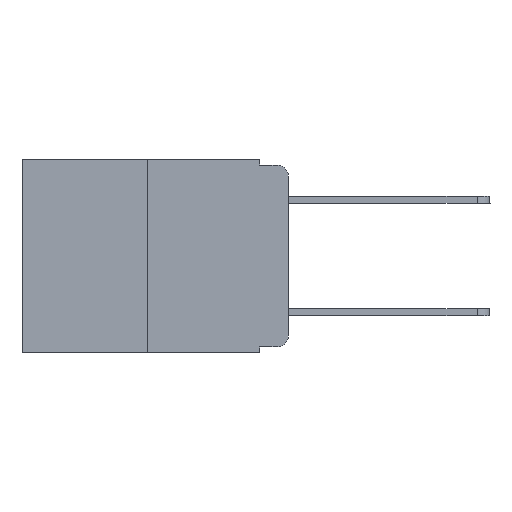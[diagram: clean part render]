
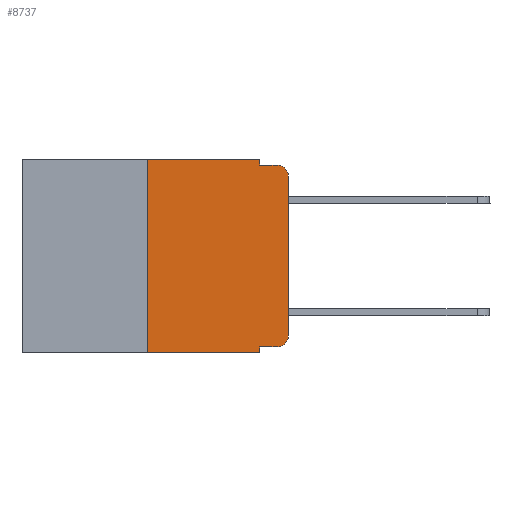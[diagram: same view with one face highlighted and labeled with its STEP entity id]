
A CAD part, left-side view. The second image highlights one B-rep face of the part: STEP entity #8737.
In plain terms, the highlighted planar face has unit normal (-1, 0, 0).
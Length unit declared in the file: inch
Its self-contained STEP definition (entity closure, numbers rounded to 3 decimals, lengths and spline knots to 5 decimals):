
#845 = VERTEX_POINT ( 'NONE', #11246 ) ;
#1171 = EDGE_CURVE ( 'NONE', #12638, #16427, #18027, .T. ) ;
#1234 = EDGE_LOOP ( 'NONE', ( #3642, #6258, #17598, #10603, #13223, #4918, #3690, #18426, #12828, #8802 ) ) ;
#1273 = VERTEX_POINT ( 'NONE', #2301 ) ;
#1366 = VECTOR ( 'NONE', #17903, 39.37008 ) ;
#1496 = DIRECTION ( 'NONE',  ( 0., -1., 0. ) ) ;
#2004 = DIRECTION ( 'NONE',  ( 0., 0., 1. ) ) ;
#2301 = CARTESIAN_POINT ( 'NONE',  ( 0., 0.051, -0.343 ) ) ;
#3559 = VECTOR ( 'NONE', #6143, 39.37008 ) ;
#3642 = ORIENTED_EDGE ( 'NONE', *, *, #10193, .T. ) ;
#3690 = ORIENTED_EDGE ( 'NONE', *, *, #9204, .T. ) ;
#3753 = DIRECTION ( 'NONE',  ( 1., 0., 0. ) ) ;
#3826 = CARTESIAN_POINT ( 'NONE',  ( 0., 0.051, -0.333 ) ) ;
#4065 = DIRECTION ( 'NONE',  ( 0., 0., 1. ) ) ;
#4355 = CARTESIAN_POINT ( 'NONE',  ( 0., 0.02, -0.333 ) ) ;
#4918 = ORIENTED_EDGE ( 'NONE', *, *, #5948, .F. ) ;
#5198 = VERTEX_POINT ( 'NONE', #15823 ) ;
#5510 = VECTOR ( 'NONE', #7941, 39.37008 ) ;
#5948 = EDGE_CURVE ( 'NONE', #6096, #845, #6166, .T. ) ;
#6059 = CARTESIAN_POINT ( 'NONE',  ( 0., 0.051, -0.01 ) ) ;
#6093 = LINE ( 'NONE', #22038, #20077 ) ;
#6096 = VERTEX_POINT ( 'NONE', #6820 ) ;
#6143 = DIRECTION ( 'NONE',  ( 0., -1., 0. ) ) ;
#6166 = LINE ( 'NONE', #13806, #19857 ) ;
#6224 = CARTESIAN_POINT ( 'NONE',  ( 0., 0.051, 0. ) ) ;
#6237 = VERTEX_POINT ( 'NONE', #18385 ) ;
#6258 = ORIENTED_EDGE ( 'NONE', *, *, #21235, .T. ) ;
#6820 = CARTESIAN_POINT ( 'NONE',  ( 0., 0.25, -0.343 ) ) ;
#7347 = VECTOR ( 'NONE', #13182, 39.37008 ) ;
#7941 = DIRECTION ( 'NONE',  ( 0., 0., -1. ) ) ;
#8374 = VERTEX_POINT ( 'NONE', #14708 ) ;
#8737 = ADVANCED_FACE ( 'NONE', ( #10487 ), #11644, .F. ) ;
#8802 = ORIENTED_EDGE ( 'NONE', *, *, #1171, .T. ) ;
#9015 = CARTESIAN_POINT ( 'NONE',  ( 0., 0.02, -0.313 ) ) ;
#9204 = EDGE_CURVE ( 'NONE', #6096, #1273, #18275, .T. ) ;
#9971 = VECTOR ( 'NONE', #1496, 39.37008 ) ;
#10018 = CARTESIAN_POINT ( 'NONE',  ( 0., 0.051, 0. ) ) ;
#10193 = EDGE_CURVE ( 'NONE', #16427, #21593, #6093, .T. ) ;
#10400 = LINE ( 'NONE', #3826, #1366 ) ;
#10487 = FACE_OUTER_BOUND ( 'NONE', #1234, .T. ) ;
#10603 = ORIENTED_EDGE ( 'NONE', *, *, #12432, .F. ) ;
#11202 = EDGE_CURVE ( 'NONE', #8374, #12638, #10400, .T. ) ;
#11246 = CARTESIAN_POINT ( 'NONE',  ( 0., 0.25, 0. ) ) ;
#11427 = CARTESIAN_POINT ( 'NONE',  ( 0., 0., -0.313 ) ) ;
#11644 = PLANE ( 'NONE',  #25113 ) ;
#12304 = DIRECTION ( 'NONE',  ( -1., 0., 0. ) ) ;
#12432 = EDGE_CURVE ( 'NONE', #24464, #6237, #25014, .T. ) ;
#12638 = VERTEX_POINT ( 'NONE', #4355 ) ;
#12828 = ORIENTED_EDGE ( 'NONE', *, *, #11202, .T. ) ;
#13182 = DIRECTION ( 'NONE',  ( 0., -1., 0. ) ) ;
#13223 = ORIENTED_EDGE ( 'NONE', *, *, #13589, .F. ) ;
#13589 = EDGE_CURVE ( 'NONE', #845, #24464, #24638, .T. ) ;
#13756 = DIRECTION ( 'NONE',  ( 0., 0., -1. ) ) ;
#13787 = CARTESIAN_POINT ( 'NONE',  ( 0., 0.02, -0.03 ) ) ;
#13806 = CARTESIAN_POINT ( 'NONE',  ( 0., 0.25, 0. ) ) ;
#14379 = AXIS2_PLACEMENT_3D ( 'NONE', #9015, #15612, #25466 ) ;
#14708 = CARTESIAN_POINT ( 'NONE',  ( 0., 0.051, -0.333 ) ) ;
#14881 = CIRCLE ( 'NONE', #17590, 0.02 ) ;
#15270 = CARTESIAN_POINT ( 'NONE',  ( 0., 0.473, 0. ) ) ;
#15560 = EDGE_CURVE ( 'NONE', #8374, #1273, #16081, .T. ) ;
#15612 = DIRECTION ( 'NONE',  ( -1., 0., 0. ) ) ;
#15823 = CARTESIAN_POINT ( 'NONE',  ( 0., 0.02, -0.01 ) ) ;
#16081 = LINE ( 'NONE', #6224, #5510 ) ;
#16427 = VERTEX_POINT ( 'NONE', #11427 ) ;
#16615 = EDGE_CURVE ( 'NONE', #6237, #5198, #18204, .T. ) ;
#17590 = AXIS2_PLACEMENT_3D ( 'NONE', #13787, #12304, #18372 ) ;
#17598 = ORIENTED_EDGE ( 'NONE', *, *, #16615, .F. ) ;
#17903 = DIRECTION ( 'NONE',  ( 0., -1., 0. ) ) ;
#18027 = CIRCLE ( 'NONE', #14379, 0.02 ) ;
#18204 = LINE ( 'NONE', #6059, #3559 ) ;
#18275 = LINE ( 'NONE', #25310, #7347 ) ;
#18372 = DIRECTION ( 'NONE',  ( 0., 0., -1. ) ) ;
#18385 = CARTESIAN_POINT ( 'NONE',  ( 0., 0.051, -0.01 ) ) ;
#18426 = ORIENTED_EDGE ( 'NONE', *, *, #15560, .F. ) ;
#19692 = VECTOR ( 'NONE', #13756, 39.37008 ) ;
#19857 = VECTOR ( 'NONE', #4065, 39.37008 ) ;
#20077 = VECTOR ( 'NONE', #2004, 39.37008 ) ;
#21235 = EDGE_CURVE ( 'NONE', #21593, #5198, #14881, .T. ) ;
#21563 = DIRECTION ( 'NONE',  ( 0., 0., -1. ) ) ;
#21593 = VERTEX_POINT ( 'NONE', #24936 ) ;
#22038 = CARTESIAN_POINT ( 'NONE',  ( 0., 0., 0. ) ) ;
#24464 = VERTEX_POINT ( 'NONE', #10018 ) ;
#24638 = LINE ( 'NONE', #15270, #9971 ) ;
#24936 = CARTESIAN_POINT ( 'NONE',  ( 0., 0., -0.03 ) ) ;
#25014 = LINE ( 'NONE', #25522, #19692 ) ;
#25113 = AXIS2_PLACEMENT_3D ( 'NONE', #25601, #3753, #21563 ) ;
#25310 = CARTESIAN_POINT ( 'NONE',  ( 0., 0.473, -0.343 ) ) ;
#25466 = DIRECTION ( 'NONE',  ( 0., 0., -1. ) ) ;
#25522 = CARTESIAN_POINT ( 'NONE',  ( 0., 0.051, 0. ) ) ;
#25601 = CARTESIAN_POINT ( 'NONE',  ( 0., 0.473, 0. ) ) ;
